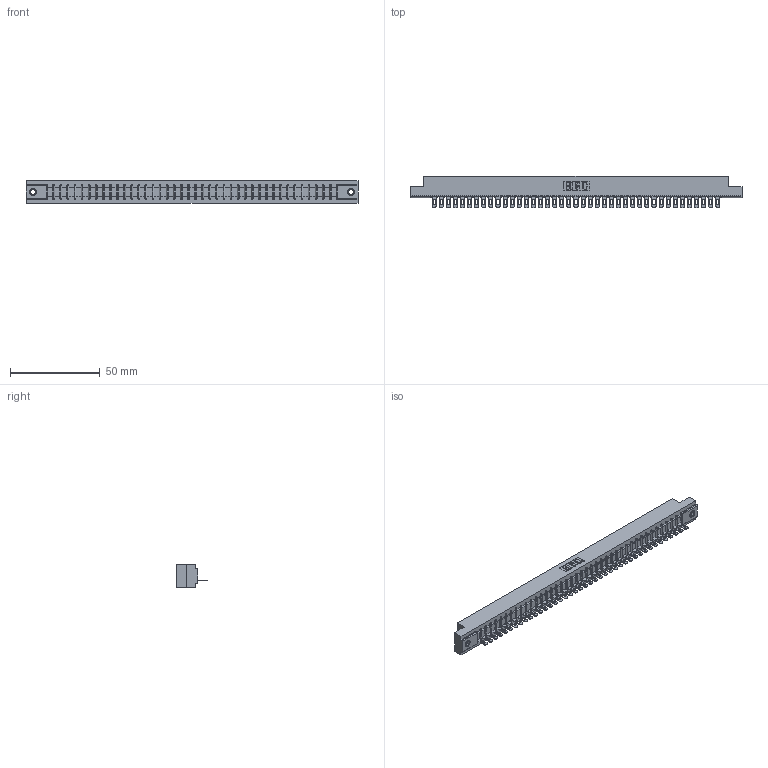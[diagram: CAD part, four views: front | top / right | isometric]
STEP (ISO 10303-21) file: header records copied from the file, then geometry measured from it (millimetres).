
FILE_DESCRIPTION (( 'STEP AP203' ), '1' );
FILE_NAME ('307-041-501-107.STEP', '2018-08-05T16:06:23', ( '' ), ( '' ), 'SwSTEP 2.0', 'SolidWorks 2016', '' );
FILE_SCHEMA (( 'CONFIG_CONTROL_DESIGN' ));
Length unit declared in the file: inch
Products named in the file (4): 307 Part_.156 Dia Mounting Holes; 307-290-002_501; 345-250-001_345-250-005-103; 307-041-501-107
Assembly tree (44 placements, depth 2):
  307-041-501-107
    307 Part_.156 Dia Mounting Holes
    307-290-002_501  x41
    345-250-001_345-250-005-103  x2
Bounding box: 185.47 x 17.42 x 12.7 mm (x, y, z)
Volume: 19862.5 mm3; surface area: 25261.7 mm2
Topology: 44 solids, 44 shells, 3336 faces, 10217 edges, 6690 vertices
Faces by surface type: plane 1906, cylinder 1330, sphere 84, cone 12, torus 4
Entity records: 37251 total; most frequent: CARTESIAN_POINT 6263, ORIENTED_EDGE 6246, DIRECTION 6099, EDGE_CURVE 3123, VECTOR 2387, LINE 2387, VERTEX_POINT 2020, AXIS2_PLACEMENT_3D 1856
